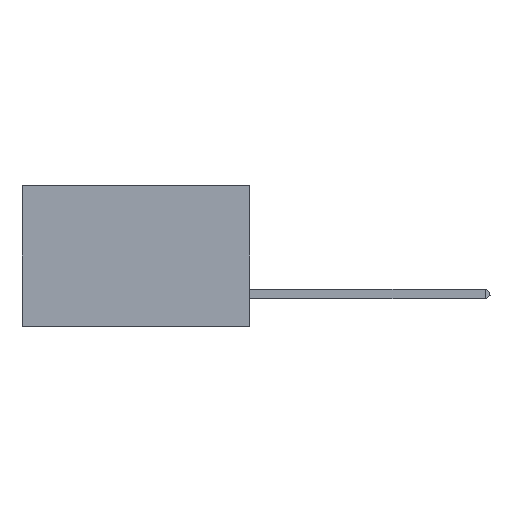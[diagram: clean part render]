
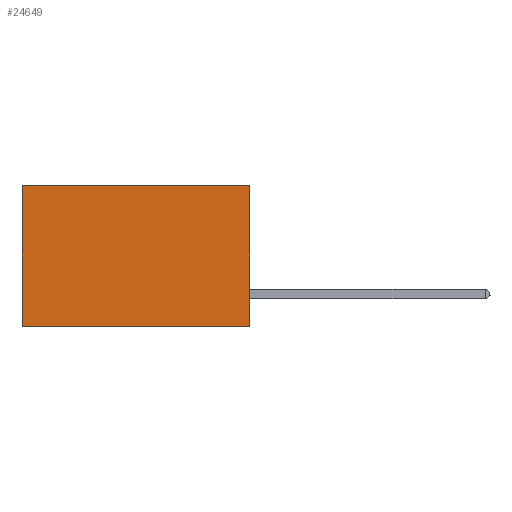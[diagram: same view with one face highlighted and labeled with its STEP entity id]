
A CAD part, left-side view. The second image highlights one B-rep face of the part: STEP entity #24649.
In plain terms, the highlighted planar face has unit normal (-1, 0, 0).
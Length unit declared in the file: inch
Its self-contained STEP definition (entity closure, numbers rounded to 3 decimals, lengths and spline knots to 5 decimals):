
#109 = LINE ( 'NONE', #5075, #18882 ) ;
#275 = DIRECTION ( 'NONE',  ( 0., 0., -1. ) ) ;
#958 = EDGE_CURVE ( 'NONE', #8870, #27041, #12353, .T. ) ;
#2585 = PLANE ( 'NONE',  #7959 ) ;
#2749 = DIRECTION ( 'NONE',  ( 0., 1., 0. ) ) ;
#2845 = FACE_OUTER_BOUND ( 'NONE', #27561, .T. ) ;
#3131 = CARTESIAN_POINT ( 'NONE',  ( 0.2875, 0., -0.37 ) ) ;
#4473 = DIRECTION ( 'NONE',  ( 0., 1., 0. ) ) ;
#4870 = VERTEX_POINT ( 'NONE', #6163 ) ;
#5075 = CARTESIAN_POINT ( 'NONE',  ( 0.2875, 0., 0. ) ) ;
#5165 = DIRECTION ( 'NONE',  ( 0., 0., -1. ) ) ;
#6163 = CARTESIAN_POINT ( 'NONE',  ( 0.2875, 0., -0.37 ) ) ;
#7167 = LINE ( 'NONE', #22480, #18103 ) ;
#7959 = AXIS2_PLACEMENT_3D ( 'NONE', #24463, #22329, #275 ) ;
#8693 = ORIENTED_EDGE ( 'NONE', *, *, #19061, .T. ) ;
#8870 = VERTEX_POINT ( 'NONE', #11536 ) ;
#9851 = LINE ( 'NONE', #3131, #25985 ) ;
#11313 = ORIENTED_EDGE ( 'NONE', *, *, #17919, .F. ) ;
#11536 = CARTESIAN_POINT ( 'NONE',  ( 0.2875, 0., 0. ) ) ;
#12353 = LINE ( 'NONE', #19513, #17177 ) ;
#13273 = CARTESIAN_POINT ( 'NONE',  ( 0.2875, 0.6, 0. ) ) ;
#14881 = EDGE_CURVE ( 'NONE', #4870, #16211, #9851, .T. ) ;
#16211 = VERTEX_POINT ( 'NONE', #26158 ) ;
#17177 = VECTOR ( 'NONE', #4473, 39.37008 ) ;
#17919 = EDGE_CURVE ( 'NONE', #8870, #4870, #109, .T. ) ;
#18103 = VECTOR ( 'NONE', #18145, 39.37008 ) ;
#18145 = DIRECTION ( 'NONE',  ( 0., 0., -1. ) ) ;
#18882 = VECTOR ( 'NONE', #5165, 39.37008 ) ;
#19061 = EDGE_CURVE ( 'NONE', #27041, #16211, #7167, .T. ) ;
#19513 = CARTESIAN_POINT ( 'NONE',  ( 0.2875, 0., 0. ) ) ;
#21932 = ORIENTED_EDGE ( 'NONE', *, *, #958, .T. ) ;
#22329 = DIRECTION ( 'NONE',  ( 1., 0., 0. ) ) ;
#22480 = CARTESIAN_POINT ( 'NONE',  ( 0.2875, 0.6, 0. ) ) ;
#24463 = CARTESIAN_POINT ( 'NONE',  ( 0.2875, 0., 0. ) ) ;
#24649 = ADVANCED_FACE ( 'NONE', ( #2845 ), #2585, .F. ) ;
#25985 = VECTOR ( 'NONE', #2749, 39.37008 ) ;
#26158 = CARTESIAN_POINT ( 'NONE',  ( 0.2875, 0.6, -0.37 ) ) ;
#27041 = VERTEX_POINT ( 'NONE', #13273 ) ;
#27561 = EDGE_LOOP ( 'NONE', ( #8693, #27778, #11313, #21932 ) ) ;
#27778 = ORIENTED_EDGE ( 'NONE', *, *, #14881, .F. ) ;
